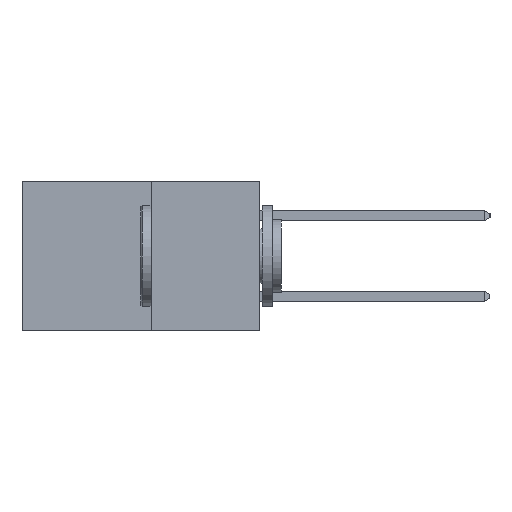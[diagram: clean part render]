
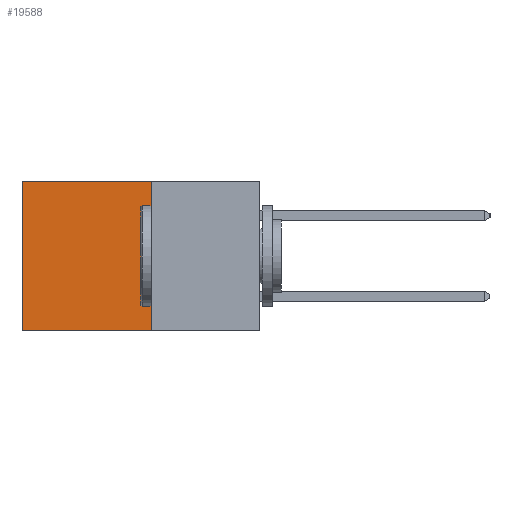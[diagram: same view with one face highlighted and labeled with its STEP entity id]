
A CAD part, left-side view. The second image highlights one B-rep face of the part: STEP entity #19588.
In plain terms, the highlighted planar face has unit normal (-1, 0, 0).
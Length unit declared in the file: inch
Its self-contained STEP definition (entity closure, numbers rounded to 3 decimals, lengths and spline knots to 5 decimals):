
#292 = DIRECTION ( 'NONE',  ( 0., 0., -1. ) ) ;
#516 = FACE_OUTER_BOUND ( 'NONE', #13668, .T. ) ;
#959 = DIRECTION ( 'NONE',  ( 0., 1., 0. ) ) ;
#1489 = ORIENTED_EDGE ( 'NONE', *, *, #17790, .T. ) ;
#1507 = CARTESIAN_POINT ( 'NONE',  ( 0.277, 0.27, -0.37 ) ) ;
#2414 = AXIS2_PLACEMENT_3D ( 'NONE', #7498, #17002, #5627 ) ;
#3487 = VERTEX_POINT ( 'NONE', #1507 ) ;
#3513 = DIRECTION ( 'NONE',  ( 0., 1., 0. ) ) ;
#4592 = CARTESIAN_POINT ( 'NONE',  ( 0.277, 0.59, 0. ) ) ;
#5125 = DIRECTION ( 'NONE',  ( 0., 0., -1. ) ) ;
#5627 = DIRECTION ( 'NONE',  ( 0., 0., -1. ) ) ;
#5749 = EDGE_CURVE ( 'NONE', #23723, #20738, #18645, .T. ) ;
#6024 = ORIENTED_EDGE ( 'NONE', *, *, #17573, .F. ) ;
#6516 = CARTESIAN_POINT ( 'NONE',  ( 0.277, 0.59, -0.37 ) ) ;
#7116 = LINE ( 'NONE', #16814, #18312 ) ;
#7293 = CARTESIAN_POINT ( 'NONE',  ( 0.277, 0.59, -0.37 ) ) ;
#7498 = CARTESIAN_POINT ( 'NONE',  ( 0.277, 0.27, -0.37 ) ) ;
#7624 = LINE ( 'NONE', #23646, #22055 ) ;
#7791 = VERTEX_POINT ( 'NONE', #19774 ) ;
#12403 = VECTOR ( 'NONE', #292, 39.37008 ) ;
#13651 = VECTOR ( 'NONE', #5125, 39.37008 ) ;
#13668 = EDGE_LOOP ( 'NONE', ( #19924, #15545, #6024, #1489 ) ) ;
#15545 = ORIENTED_EDGE ( 'NONE', *, *, #22156, .F. ) ;
#16814 = CARTESIAN_POINT ( 'NONE',  ( 0.277, 0.27, -0.37 ) ) ;
#16838 = PLANE ( 'NONE',  #2414 ) ;
#17002 = DIRECTION ( 'NONE',  ( 1., 0., 0. ) ) ;
#17573 = EDGE_CURVE ( 'NONE', #7791, #3487, #22345, .T. ) ;
#17790 = EDGE_CURVE ( 'NONE', #7791, #23723, #7624, .T. ) ;
#18312 = VECTOR ( 'NONE', #3513, 39.37008 ) ;
#18645 = LINE ( 'NONE', #6516, #13651 ) ;
#19588 = ADVANCED_FACE ( 'NONE', ( #516 ), #16838, .F. ) ;
#19774 = CARTESIAN_POINT ( 'NONE',  ( 0.277, 0.27, 0. ) ) ;
#19924 = ORIENTED_EDGE ( 'NONE', *, *, #5749, .T. ) ;
#20738 = VERTEX_POINT ( 'NONE', #7293 ) ;
#22055 = VECTOR ( 'NONE', #959, 39.37008 ) ;
#22156 = EDGE_CURVE ( 'NONE', #3487, #20738, #7116, .T. ) ;
#22345 = LINE ( 'NONE', #22992, #12403 ) ;
#22992 = CARTESIAN_POINT ( 'NONE',  ( 0.277, 0.27, -0.37 ) ) ;
#23646 = CARTESIAN_POINT ( 'NONE',  ( 0.277, 0.27, 0. ) ) ;
#23723 = VERTEX_POINT ( 'NONE', #4592 ) ;
